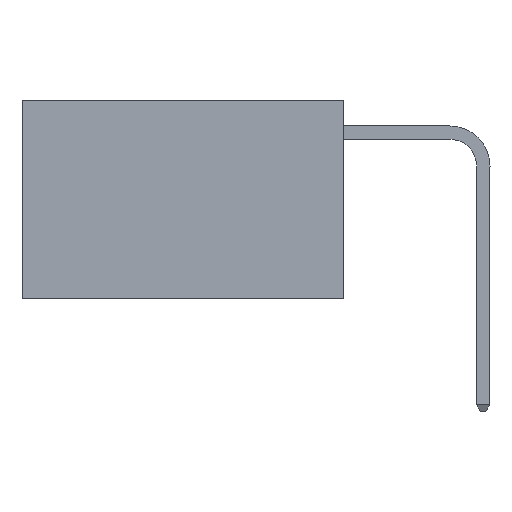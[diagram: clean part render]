
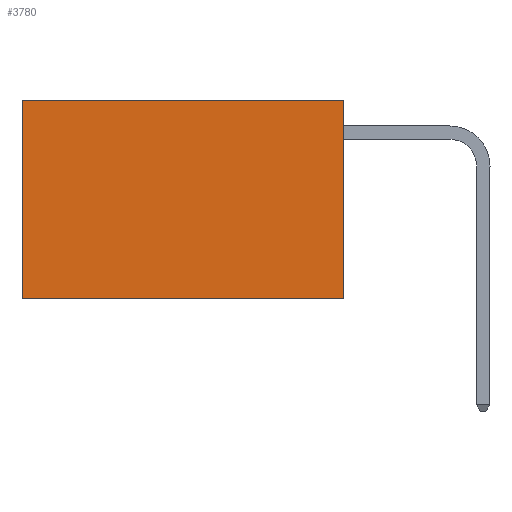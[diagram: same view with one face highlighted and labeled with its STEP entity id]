
A CAD part, left-side view. The second image highlights one B-rep face of the part: STEP entity #3780.
In plain terms, the highlighted planar face has unit normal (-1, 0, 0).
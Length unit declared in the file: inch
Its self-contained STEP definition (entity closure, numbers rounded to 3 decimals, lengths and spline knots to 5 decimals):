
#297 = CARTESIAN_POINT ( 'NONE',  ( 0.2625, 0.6, 0. ) ) ;
#556 = EDGE_CURVE ( 'NONE', #7921, #7830, #9139, .T. ) ;
#1841 = ORIENTED_EDGE ( 'NONE', *, *, #9598, .F. ) ;
#1998 = CARTESIAN_POINT ( 'NONE',  ( 0.2625, 0., 0. ) ) ;
#2426 = DIRECTION ( 'NONE',  ( 0., 0., -1. ) ) ;
#2442 = DIRECTION ( 'NONE',  ( 1., 0., 0. ) ) ;
#2494 = PLANE ( 'NONE',  #5881 ) ;
#2623 = CARTESIAN_POINT ( 'NONE',  ( 0.2625, 0., 0. ) ) ;
#2726 = FACE_OUTER_BOUND ( 'NONE', #8416, .T. ) ;
#2765 = CARTESIAN_POINT ( 'NONE',  ( 0.2625, 0., -0.37 ) ) ;
#2895 = VECTOR ( 'NONE', #3982, 39.37008 ) ;
#3259 = VERTEX_POINT ( 'NONE', #297 ) ;
#3371 = CARTESIAN_POINT ( 'NONE',  ( 0.2625, 0.6, -0.37 ) ) ;
#3780 = ADVANCED_FACE ( 'NONE', ( #2726 ), #2494, .F. ) ;
#3982 = DIRECTION ( 'NONE',  ( 0., 0., -1. ) ) ;
#4538 = ORIENTED_EDGE ( 'NONE', *, *, #8918, .T. ) ;
#5168 = DIRECTION ( 'NONE',  ( 0., 0., -1. ) ) ;
#5255 = LINE ( 'NONE', #8876, #2895 ) ;
#5881 = AXIS2_PLACEMENT_3D ( 'NONE', #2623, #2442, #2426 ) ;
#6255 = CARTESIAN_POINT ( 'NONE',  ( 0.2625, 0., -0.37 ) ) ;
#7068 = VECTOR ( 'NONE', #5168, 39.37008 ) ;
#7254 = DIRECTION ( 'NONE',  ( 0., 1., 0. ) ) ;
#7261 = VECTOR ( 'NONE', #7254, 39.37008 ) ;
#7830 = VERTEX_POINT ( 'NONE', #2765 ) ;
#7857 = VECTOR ( 'NONE', #8649, 39.37008 ) ;
#7921 = VERTEX_POINT ( 'NONE', #1998 ) ;
#7990 = CARTESIAN_POINT ( 'NONE',  ( 0.2625, 0., 0. ) ) ;
#8085 = LINE ( 'NONE', #6255, #7857 ) ;
#8132 = EDGE_CURVE ( 'NONE', #3259, #8388, #5255, .T. ) ;
#8388 = VERTEX_POINT ( 'NONE', #3371 ) ;
#8416 = EDGE_LOOP ( 'NONE', ( #10379, #1841, #8563, #4538 ) ) ;
#8563 = ORIENTED_EDGE ( 'NONE', *, *, #556, .F. ) ;
#8649 = DIRECTION ( 'NONE',  ( 0., 1., 0. ) ) ;
#8876 = CARTESIAN_POINT ( 'NONE',  ( 0.2625, 0.6, 0. ) ) ;
#8918 = EDGE_CURVE ( 'NONE', #7921, #3259, #9357, .T. ) ;
#9139 = LINE ( 'NONE', #9819, #7068 ) ;
#9357 = LINE ( 'NONE', #7990, #7261 ) ;
#9598 = EDGE_CURVE ( 'NONE', #7830, #8388, #8085, .T. ) ;
#9819 = CARTESIAN_POINT ( 'NONE',  ( 0.2625, 0., 0. ) ) ;
#10379 = ORIENTED_EDGE ( 'NONE', *, *, #8132, .T. ) ;
